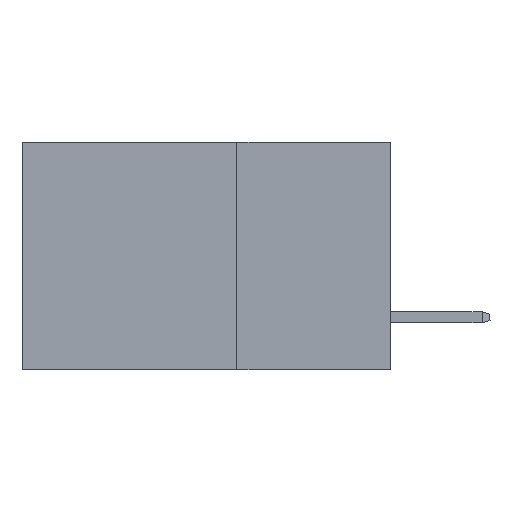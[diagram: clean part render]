
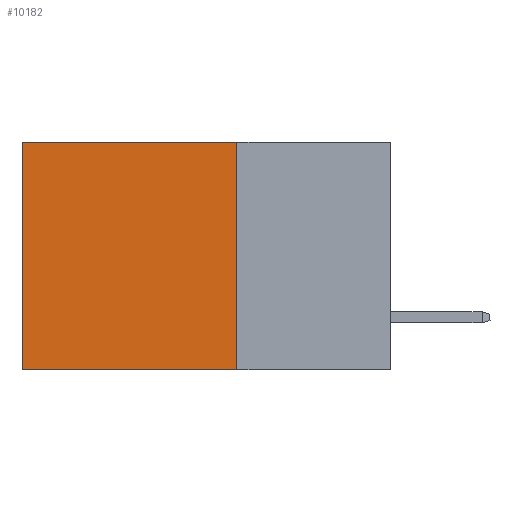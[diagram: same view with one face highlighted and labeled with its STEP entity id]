
A CAD part, left-side view. The second image highlights one B-rep face of the part: STEP entity #10182.
In plain terms, the highlighted planar face has unit normal (-1, 0, 0).
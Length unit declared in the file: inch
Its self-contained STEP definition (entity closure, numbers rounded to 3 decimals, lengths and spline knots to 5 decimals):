
#1005 = VERTEX_POINT ( 'NONE', #9961 ) ;
#1620 = CARTESIAN_POINT ( 'NONE',  ( 0.2875, 0.6, -0.37 ) ) ;
#1680 = CARTESIAN_POINT ( 'NONE',  ( 0.2875, 0.6, 0. ) ) ;
#2364 = LINE ( 'NONE', #1680, #6440 ) ;
#2517 = CARTESIAN_POINT ( 'NONE',  ( 0.2875, 0.25, 0. ) ) ;
#2721 = PLANE ( 'NONE',  #4915 ) ;
#2796 = ORIENTED_EDGE ( 'NONE', *, *, #3020, .F. ) ;
#2929 = CARTESIAN_POINT ( 'NONE',  ( 0.2875, 0.6, 0. ) ) ;
#3020 = EDGE_CURVE ( 'NONE', #7528, #1005, #3677, .T. ) ;
#3550 = DIRECTION ( 'NONE',  ( 1., 0., 0. ) ) ;
#3646 = LINE ( 'NONE', #6988, #9549 ) ;
#3677 = LINE ( 'NONE', #9324, #7698 ) ;
#4069 = EDGE_CURVE ( 'NONE', #8496, #9447, #2364, .T. ) ;
#4083 = LINE ( 'NONE', #2517, #7587 ) ;
#4195 = DIRECTION ( 'NONE',  ( 0., 0., -1. ) ) ;
#4215 = ORIENTED_EDGE ( 'NONE', *, *, #4393, .F. ) ;
#4393 = EDGE_CURVE ( 'NONE', #1005, #9447, #3646, .T. ) ;
#4915 = AXIS2_PLACEMENT_3D ( 'NONE', #5123, #3550, #9174 ) ;
#5123 = CARTESIAN_POINT ( 'NONE',  ( 0.2875, 0.25, 0. ) ) ;
#5787 = EDGE_CURVE ( 'NONE', #7528, #8496, #4083, .T. ) ;
#6130 = EDGE_LOOP ( 'NONE', ( #9845, #4215, #2796, #7835 ) ) ;
#6184 = DIRECTION ( 'NONE',  ( 0., 1., 0. ) ) ;
#6440 = VECTOR ( 'NONE', #4195, 39.37008 ) ;
#6988 = CARTESIAN_POINT ( 'NONE',  ( 0.2875, 0.25, -0.37 ) ) ;
#7317 = CARTESIAN_POINT ( 'NONE',  ( 0.2875, 0.25, 0. ) ) ;
#7350 = DIRECTION ( 'NONE',  ( 0., 1., 0. ) ) ;
#7372 = FACE_OUTER_BOUND ( 'NONE', #6130, .T. ) ;
#7528 = VERTEX_POINT ( 'NONE', #7317 ) ;
#7587 = VECTOR ( 'NONE', #7350, 39.37008 ) ;
#7698 = VECTOR ( 'NONE', #8528, 39.37008 ) ;
#7835 = ORIENTED_EDGE ( 'NONE', *, *, #5787, .T. ) ;
#8496 = VERTEX_POINT ( 'NONE', #2929 ) ;
#8528 = DIRECTION ( 'NONE',  ( 0., 0., -1. ) ) ;
#9174 = DIRECTION ( 'NONE',  ( 0., 0., -1. ) ) ;
#9324 = CARTESIAN_POINT ( 'NONE',  ( 0.2875, 0.25, 0. ) ) ;
#9447 = VERTEX_POINT ( 'NONE', #1620 ) ;
#9549 = VECTOR ( 'NONE', #6184, 39.37008 ) ;
#9845 = ORIENTED_EDGE ( 'NONE', *, *, #4069, .T. ) ;
#9961 = CARTESIAN_POINT ( 'NONE',  ( 0.2875, 0.25, -0.37 ) ) ;
#10182 = ADVANCED_FACE ( 'NONE', ( #7372 ), #2721, .F. ) ;
